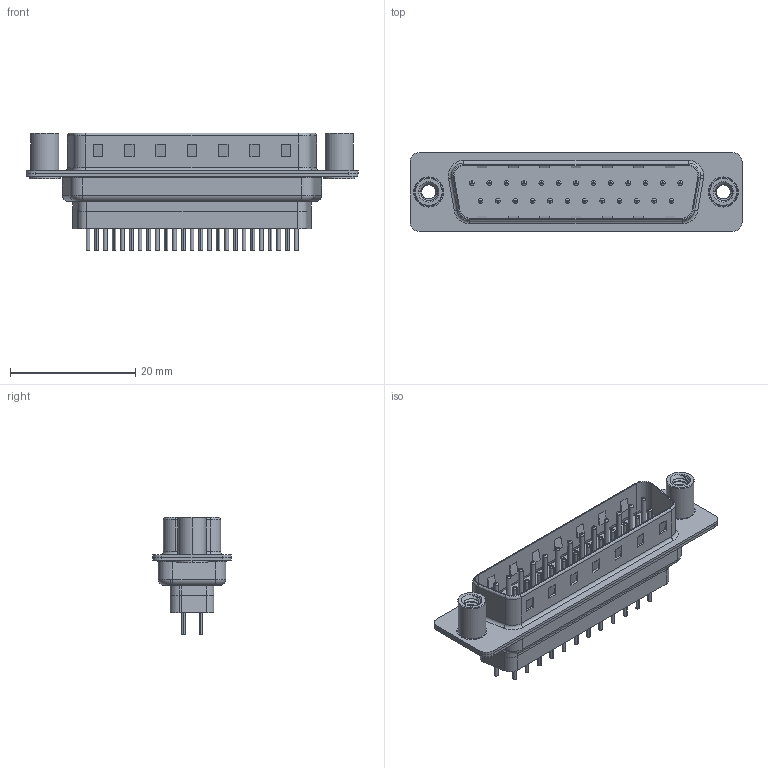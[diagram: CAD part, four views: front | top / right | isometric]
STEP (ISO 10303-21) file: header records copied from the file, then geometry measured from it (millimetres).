
FILE_DESCRIPTION (( 'STEP AP203' ), '1' );
FILE_NAME ('627-025-228-268.STEP', '2020-07-21T16:49:26', ( '' ), ( '' ), 'SwSTEP 2.0', 'SolidWorks 2020', '' );
FILE_SCHEMA (( 'CONFIG_CONTROL_DESIGN' ));
Length unit declared in the file: millimetre
Products named in the file (7): 627 Shell Rear_25 Contacts; 627 Shell Front_25 Contacts; 627 Contact Row 1_28L; 627-025-228-268; 627 Contact Row 2_28L; 627 4-40 Threaded Standoff; 627 Housing_25 FF
Assembly tree (30 placements, depth 2):
  627-025-228-268
    627 Housing_25 FF
    627 Shell Front_25 Contacts
    627 Shell Rear_25 Contacts
    627 Contact Row 1_28L  x13
    627 Contact Row 2_28L  x12
    627 4-40 Threaded Standoff  x2
Bounding box: 53 x 12.6 x 18.8 mm (x, y, z)
Volume: 3341.2 mm3; surface area: 9119.1 mm2
Topology: 31 solids, 31 shells, 2921 faces, 7651 edges, 4755 vertices
Faces by surface type: cylinder 1145, plane 779, torus 725, cone 266, bspline 6
Entity records: 28035 total; most frequent: CARTESIAN_POINT 6493, DIRECTION 4495, ORIENTED_EDGE 4038, EDGE_CURVE 2019, AXIS2_PLACEMENT_3D 1780, VERTEX_POINT 1292, EDGE_LOOP 1003, CIRCLE 949
